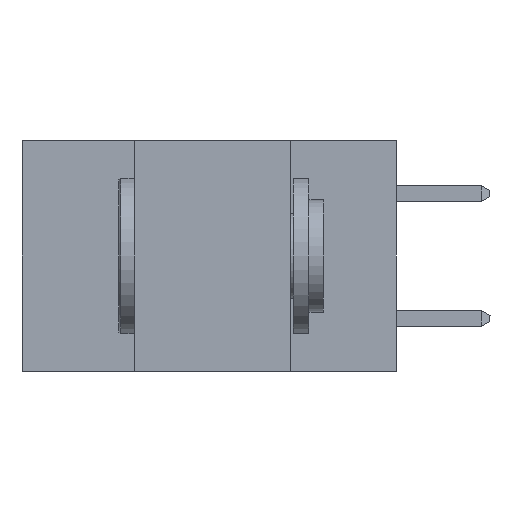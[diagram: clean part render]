
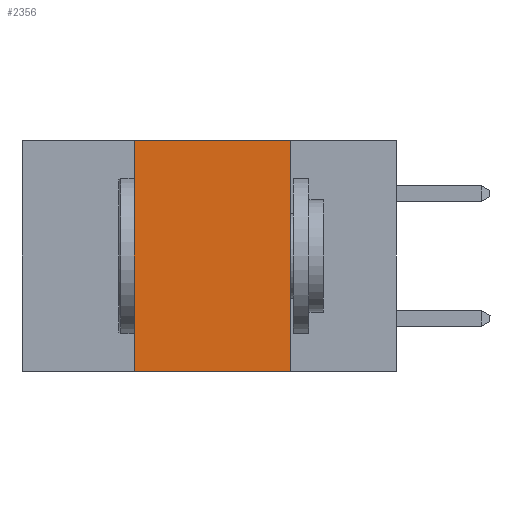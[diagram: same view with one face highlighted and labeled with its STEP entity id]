
A CAD part, left-side view. The second image highlights one B-rep face of the part: STEP entity #2356.
In plain terms, the highlighted planar face has unit normal (-1, 0, 0).
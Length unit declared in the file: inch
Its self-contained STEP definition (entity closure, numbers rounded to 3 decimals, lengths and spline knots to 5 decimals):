
#1272 = FACE_OUTER_BOUND ( 'NONE', #6713, .T. ) ;
#1321 = VERTEX_POINT ( 'NONE', #1550 ) ;
#1550 = CARTESIAN_POINT ( 'NONE',  ( 0., 0.17, -0.37 ) ) ;
#1948 = EDGE_CURVE ( 'NONE', #10276, #1321, #10688, .T. ) ;
#2333 = LINE ( 'NONE', #9863, #7246 ) ;
#2356 = ADVANCED_FACE ( 'NONE', ( #1272 ), #7552, .F. ) ;
#2406 = ORIENTED_EDGE ( 'NONE', *, *, #1948, .T. ) ;
#3215 = EDGE_CURVE ( 'NONE', #5796, #5019, #2333, .T. ) ;
#3338 = CARTESIAN_POINT ( 'NONE',  ( 0., 0.42, -0.37 ) ) ;
#3459 = VECTOR ( 'NONE', #11695, 39.37008 ) ;
#4370 = DIRECTION ( 'NONE',  ( 0., 0., 1. ) ) ;
#4811 = ORIENTED_EDGE ( 'NONE', *, *, #3215, .F. ) ;
#5019 = VERTEX_POINT ( 'NONE', #10368 ) ;
#5403 = CARTESIAN_POINT ( 'NONE',  ( 0., 0.6, 0. ) ) ;
#5796 = VERTEX_POINT ( 'NONE', #7112 ) ;
#6631 = CARTESIAN_POINT ( 'NONE',  ( 0., 0.42, -0.37 ) ) ;
#6713 = EDGE_LOOP ( 'NONE', ( #9478, #4811, #9761, #2406 ) ) ;
#7112 = CARTESIAN_POINT ( 'NONE',  ( 0., 0.42, 0. ) ) ;
#7246 = VECTOR ( 'NONE', #9142, 39.37008 ) ;
#7550 = EDGE_CURVE ( 'NONE', #10276, #5796, #12366, .T. ) ;
#7552 = PLANE ( 'NONE',  #8226 ) ;
#8226 = AXIS2_PLACEMENT_3D ( 'NONE', #5403, #8506, #8490 ) ;
#8330 = DIRECTION ( 'NONE',  ( 0., 0., -1. ) ) ;
#8490 = DIRECTION ( 'NONE',  ( 0., 0., -1. ) ) ;
#8506 = DIRECTION ( 'NONE',  ( 1., 0., 0. ) ) ;
#8547 = EDGE_CURVE ( 'NONE', #5019, #1321, #12340, .T. ) ;
#8562 = CARTESIAN_POINT ( 'NONE',  ( 0., 0.6, -0.37 ) ) ;
#9142 = DIRECTION ( 'NONE',  ( 0., -1., 0. ) ) ;
#9478 = ORIENTED_EDGE ( 'NONE', *, *, #8547, .F. ) ;
#9702 = VECTOR ( 'NONE', #8330, 39.37008 ) ;
#9726 = VECTOR ( 'NONE', #4370, 39.37008 ) ;
#9761 = ORIENTED_EDGE ( 'NONE', *, *, #7550, .F. ) ;
#9863 = CARTESIAN_POINT ( 'NONE',  ( 0., 0.6, 0. ) ) ;
#10276 = VERTEX_POINT ( 'NONE', #6631 ) ;
#10368 = CARTESIAN_POINT ( 'NONE',  ( 0., 0.17, 0. ) ) ;
#10688 = LINE ( 'NONE', #8562, #3459 ) ;
#11695 = DIRECTION ( 'NONE',  ( 0., -1., 0. ) ) ;
#11909 = CARTESIAN_POINT ( 'NONE',  ( 0., 0.17, -0.37 ) ) ;
#12340 = LINE ( 'NONE', #11909, #9702 ) ;
#12366 = LINE ( 'NONE', #3338, #9726 ) ;
